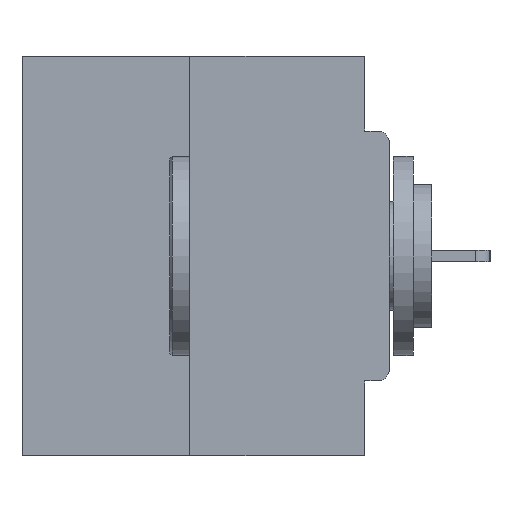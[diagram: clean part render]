
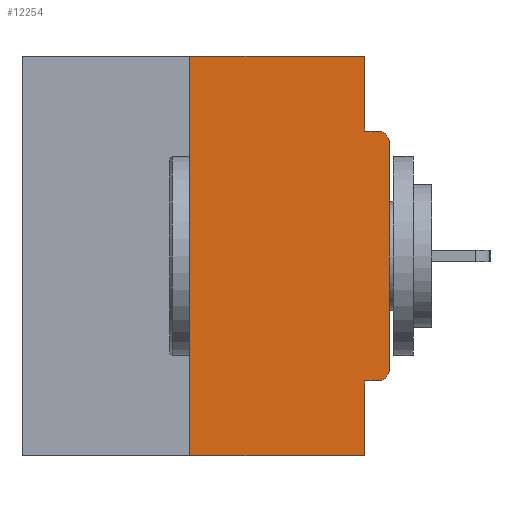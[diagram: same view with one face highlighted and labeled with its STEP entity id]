
A CAD part, left-side view. The second image highlights one B-rep face of the part: STEP entity #12254.
In plain terms, the highlighted planar face has unit normal (-1, 0, 0).
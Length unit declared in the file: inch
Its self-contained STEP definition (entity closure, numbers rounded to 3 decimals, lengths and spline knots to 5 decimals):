
#398 = EDGE_LOOP ( 'NONE', ( #24928, #20048, #15186, #3648, #30140, #25311, #14057, #9100, #29779, #572 ) ) ;
#572 = ORIENTED_EDGE ( 'NONE', *, *, #12108, .F. ) ;
#889 = CARTESIAN_POINT ( 'NONE',  ( 0., 0.015, -0.0935 ) ) ;
#1066 = DIRECTION ( 'NONE',  ( 0., 0., 1. ) ) ;
#1644 = VECTOR ( 'NONE', #31329, 39.37008 ) ;
#1975 = CARTESIAN_POINT ( 'NONE',  ( 0., 0.031, 0. ) ) ;
#2141 = LINE ( 'NONE', #12987, #20814 ) ;
#2634 = LINE ( 'NONE', #9406, #21318 ) ;
#2663 = EDGE_CURVE ( 'NONE', #4205, #27961, #17346, .T. ) ;
#2885 = EDGE_CURVE ( 'NONE', #27492, #23751, #18256, .T. ) ;
#3005 = CARTESIAN_POINT ( 'NONE',  ( 0., 0.25, 0. ) ) ;
#3344 = EDGE_CURVE ( 'NONE', #22383, #13011, #2141, .T. ) ;
#3378 = CARTESIAN_POINT ( 'NONE',  ( 0., 0.031, -0.5 ) ) ;
#3614 = VECTOR ( 'NONE', #1066, 39.37008 ) ;
#3648 = ORIENTED_EDGE ( 'NONE', *, *, #7279, .F. ) ;
#4205 = VERTEX_POINT ( 'NONE', #7722 ) ;
#4500 = DIRECTION ( 'NONE',  ( 0., 0., -1. ) ) ;
#4606 = PLANE ( 'NONE',  #20332 ) ;
#4920 = EDGE_CURVE ( 'NONE', #29360, #27492, #21102, .T. ) ;
#6552 = DIRECTION ( 'NONE',  ( 0., 0., -1. ) ) ;
#6848 = CARTESIAN_POINT ( 'NONE',  ( 0., 0., -0.1085 ) ) ;
#7088 = DIRECTION ( 'NONE',  ( 0., 0., -1. ) ) ;
#7279 = EDGE_CURVE ( 'NONE', #22198, #11650, #25450, .T. ) ;
#7659 = DIRECTION ( 'NONE',  ( -1., 0., 0. ) ) ;
#7722 = CARTESIAN_POINT ( 'NONE',  ( 0., 0.015, -0.4065 ) ) ;
#8297 = VERTEX_POINT ( 'NONE', #6848 ) ;
#9100 = ORIENTED_EDGE ( 'NONE', *, *, #11775, .T. ) ;
#9238 = DIRECTION ( 'NONE',  ( 0., -1., 0. ) ) ;
#9406 = CARTESIAN_POINT ( 'NONE',  ( 0., 0.46, -0.5 ) ) ;
#10212 = LINE ( 'NONE', #23013, #3614 ) ;
#11458 = AXIS2_PLACEMENT_3D ( 'NONE', #24455, #31201, #29970 ) ;
#11650 = VERTEX_POINT ( 'NONE', #28861 ) ;
#11775 = EDGE_CURVE ( 'NONE', #8297, #13011, #20571, .T. ) ;
#12108 = EDGE_CURVE ( 'NONE', #23751, #22383, #17192, .T. ) ;
#12203 = EDGE_CURVE ( 'NONE', #29360, #11650, #2634, .T. ) ;
#12254 = ADVANCED_FACE ( 'NONE', ( #19809 ), #4606, .F. ) ;
#12522 = CARTESIAN_POINT ( 'NONE',  ( 0., 0., -0.4065 ) ) ;
#12987 = CARTESIAN_POINT ( 'NONE',  ( 0., 0., -0.0935 ) ) ;
#13011 = VERTEX_POINT ( 'NONE', #889 ) ;
#13363 = CARTESIAN_POINT ( 'NONE',  ( 0., 0.031, -0.0935 ) ) ;
#13557 = DIRECTION ( 'NONE',  ( 0., -1., 0. ) ) ;
#13856 = CARTESIAN_POINT ( 'NONE',  ( 0., 0.25, -0.5 ) ) ;
#14057 = ORIENTED_EDGE ( 'NONE', *, *, #25768, .T. ) ;
#15134 = VECTOR ( 'NONE', #26898, 39.37008 ) ;
#15186 = ORIENTED_EDGE ( 'NONE', *, *, #12203, .T. ) ;
#15400 = CARTESIAN_POINT ( 'NONE',  ( 0., 0., -0.3915 ) ) ;
#17192 = LINE ( 'NONE', #21115, #23574 ) ;
#17346 = CIRCLE ( 'NONE', #11458, 0.015 ) ;
#18256 = LINE ( 'NONE', #27791, #23879 ) ;
#19034 = DIRECTION ( 'NONE',  ( 0., -1., 0. ) ) ;
#19809 = FACE_OUTER_BOUND ( 'NONE', #398, .T. ) ;
#20048 = ORIENTED_EDGE ( 'NONE', *, *, #4920, .F. ) ;
#20332 = AXIS2_PLACEMENT_3D ( 'NONE', #30990, #21635, #7088 ) ;
#20571 = CIRCLE ( 'NONE', #21538, 0.015 ) ;
#20738 = LINE ( 'NONE', #12522, #15134 ) ;
#20814 = VECTOR ( 'NONE', #13557, 39.37008 ) ;
#20975 = CARTESIAN_POINT ( 'NONE',  ( 0., 0.25, 0. ) ) ;
#21102 = LINE ( 'NONE', #3005, #1644 ) ;
#21115 = CARTESIAN_POINT ( 'NONE',  ( 0., 0.031, 0. ) ) ;
#21318 = VECTOR ( 'NONE', #19034, 39.37008 ) ;
#21538 = AXIS2_PLACEMENT_3D ( 'NONE', #22190, #7659, #24605 ) ;
#21635 = DIRECTION ( 'NONE',  ( 1., 0., 0. ) ) ;
#22190 = CARTESIAN_POINT ( 'NONE',  ( 0., 0.015, -0.1085 ) ) ;
#22198 = VERTEX_POINT ( 'NONE', #26992 ) ;
#22383 = VERTEX_POINT ( 'NONE', #13363 ) ;
#23013 = CARTESIAN_POINT ( 'NONE',  ( 0., 0., 0. ) ) ;
#23574 = VECTOR ( 'NONE', #6552, 39.37008 ) ;
#23751 = VERTEX_POINT ( 'NONE', #1975 ) ;
#23879 = VECTOR ( 'NONE', #9238, 39.37008 ) ;
#24455 = CARTESIAN_POINT ( 'NONE',  ( 0., 0.015, -0.3915 ) ) ;
#24605 = DIRECTION ( 'NONE',  ( 0., 0., -1. ) ) ;
#24928 = ORIENTED_EDGE ( 'NONE', *, *, #2885, .F. ) ;
#25311 = ORIENTED_EDGE ( 'NONE', *, *, #2663, .T. ) ;
#25450 = LINE ( 'NONE', #3378, #26210 ) ;
#25768 = EDGE_CURVE ( 'NONE', #27961, #8297, #10212, .T. ) ;
#26210 = VECTOR ( 'NONE', #4500, 39.37008 ) ;
#26898 = DIRECTION ( 'NONE',  ( 0., 1., 0. ) ) ;
#26992 = CARTESIAN_POINT ( 'NONE',  ( 0., 0.031, -0.4065 ) ) ;
#27492 = VERTEX_POINT ( 'NONE', #20975 ) ;
#27791 = CARTESIAN_POINT ( 'NONE',  ( 0., 0.46, 0. ) ) ;
#27961 = VERTEX_POINT ( 'NONE', #15400 ) ;
#28484 = EDGE_CURVE ( 'NONE', #4205, #22198, #20738, .T. ) ;
#28861 = CARTESIAN_POINT ( 'NONE',  ( 0., 0.031, -0.5 ) ) ;
#29360 = VERTEX_POINT ( 'NONE', #13856 ) ;
#29779 = ORIENTED_EDGE ( 'NONE', *, *, #3344, .F. ) ;
#29970 = DIRECTION ( 'NONE',  ( 0., 0., -1. ) ) ;
#30140 = ORIENTED_EDGE ( 'NONE', *, *, #28484, .F. ) ;
#30990 = CARTESIAN_POINT ( 'NONE',  ( 0., 0.46, 0. ) ) ;
#31201 = DIRECTION ( 'NONE',  ( -1., 0., 0. ) ) ;
#31329 = DIRECTION ( 'NONE',  ( 0., 0., 1. ) ) ;
